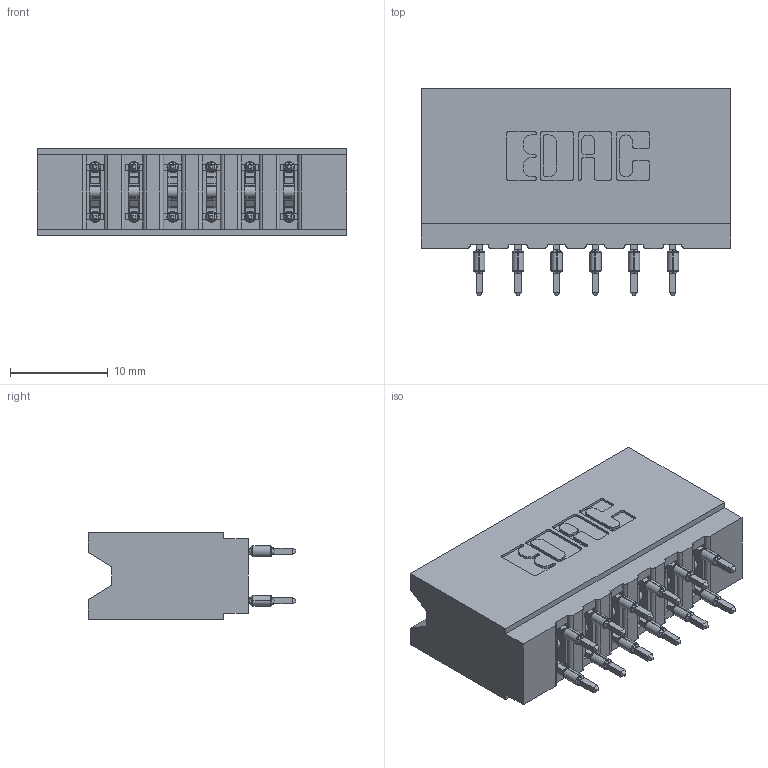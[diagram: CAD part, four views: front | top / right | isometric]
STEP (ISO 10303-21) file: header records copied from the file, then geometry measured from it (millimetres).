
FILE_DESCRIPTION (( 'STEP AP203' ), '1' );
FILE_NAME ('737-012-560-206.STEP', '2026-03-05T21:12:33', ( '' ), ( '' ), 'SwSTEP 2.0', 'SolidWorks 2023', '' );
FILE_SCHEMA (( 'CONFIG_CONTROL_DESIGN' ));
Length unit declared in the file: millimetre
Products named in the file (3): 745-292-001_560; 737 Part_Insulator Option - 06; 737-012-560-206
Assembly tree (13 placements, depth 2):
  737-012-560-206
    737 Part_Insulator Option - 06
    745-292-001_560  x12
Bounding box: 31.65 x 21.22 x 8.89 mm (x, y, z)
Volume: 3320.2 mm3; surface area: 4608 mm2
Topology: 13 solids, 13 shells, 1283 faces, 3509 edges, 2234 vertices
Faces by surface type: plane 673, cylinder 298, bspline 240, torus 72
Entity records: 15524 total; most frequent: CARTESIAN_POINT 3210, ORIENTED_EDGE 2574, DIRECTION 2283, EDGE_CURVE 1287, VECTOR 1061, LINE 1061, VERTEX_POINT 826, AXIS2_PLACEMENT_3D 611
